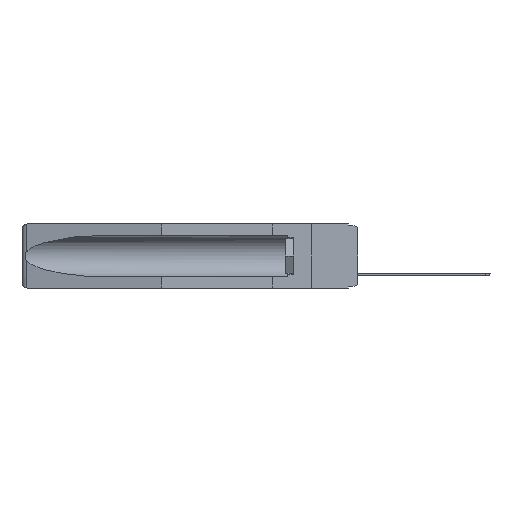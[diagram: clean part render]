
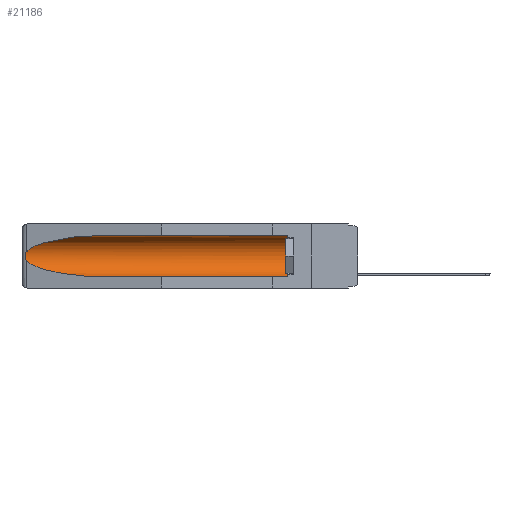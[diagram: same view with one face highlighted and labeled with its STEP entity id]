
A CAD part, left-side view. The second image highlights one B-rep face of the part: STEP entity #21186.
In plain terms, the highlighted cylindrical face has radius 2.857 mm (diameter 5.715 mm), a partial arc.
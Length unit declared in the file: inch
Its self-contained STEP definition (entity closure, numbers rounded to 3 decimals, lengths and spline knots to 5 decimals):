
#481 = CIRCLE ( 'NONE', #21289, 0.1125 ) ;
#1077 = DIRECTION ( 'NONE',  ( 0., 1., 0. ) ) ;
#1328 = DIRECTION ( 'NONE',  ( 0., 0., 1. ) ) ;
#1434 = VECTOR ( 'NONE', #1077, 39.37008 ) ;
#1686 = EDGE_CURVE ( 'NONE', #8892, #21589, #19231, .T. ) ;
#2324 = CARTESIAN_POINT ( 'NONE',  ( 0.155, 0.126, -0.284 ) ) ;
#2715 = DIRECTION ( 'NONE',  ( 0., 1., 0. ) ) ;
#2845 = CARTESIAN_POINT ( 'NONE',  ( 0.26597, 1.52961, -0.15275 ) ) ;
#3074 = CARTESIAN_POINT ( 'NONE',  ( 0.26537, 1.52718, -0.19328 ) ) ;
#3083 = CARTESIAN_POINT ( 'NONE',  ( 0.2673, 1.53269, -0.17917 ) ) ;
#3237 = EDGE_CURVE ( 'NONE', #3274, #9180, #11163, .T. ) ;
#3274 = VERTEX_POINT ( 'NONE', #3074 ) ;
#3416 = CARTESIAN_POINT ( 'NONE',  ( 0.26537, 1.52718, -0.14972 ) ) ;
#4230 = ORIENTED_EDGE ( 'NONE', *, *, #17384, .F. ) ;
#4525 = DIRECTION ( 'NONE',  ( 0., 0., 1. ) ) ;
#4943 = CYLINDRICAL_SURFACE ( 'NONE', #17287, 0.1125 ) ;
#5254 = FACE_OUTER_BOUND ( 'NONE', #5473, .T. ) ;
#5473 = EDGE_LOOP ( 'NONE', ( #9655, #9123, #10495, #4230, #18955, #6420 ) ) ;
#5537 = CARTESIAN_POINT ( 'NONE',  ( 0.155, -0.30754, -0.059 ) ) ;
#5912 = EDGE_CURVE ( 'NONE', #6770, #3274, #7760, .T. ) ;
#6420 = ORIENTED_EDGE ( 'NONE', *, *, #1686, .T. ) ;
#6770 = VERTEX_POINT ( 'NONE', #9523 ) ;
#7050 =( BOUNDED_CURVE ( )  B_SPLINE_CURVE ( 3, ( #15745, #17466, #19230, #3416 ),
 .UNSPECIFIED., .F., .F. ) 
 B_SPLINE_CURVE_WITH_KNOTS ( ( 4, 4 ),
 ( 4.71239, 6.08839 ),
 .UNSPECIFIED. ) 
 CURVE ( )  GEOMETRIC_REPRESENTATION_ITEM ( )  RATIONAL_B_SPLINE_CURVE ( ( 1., 0.848, 0.848, 1. ) ) 
 REPRESENTATION_ITEM ( '' )  );
#7760 = B_SPLINE_CURVE_WITH_KNOTS ( 'NONE', 3,
 ( #9876, #2845, #8389, #13644, #20749, #15331, #3083, #22242, #18968, #11844 ),
 .UNSPECIFIED., .F., .F.,
 ( 4, 2, 2, 2, 4 ),
 ( 0., 0.00029, 0.00058, 0.00087, 0.00117 ),
 .UNSPECIFIED. ) ;
#8104 = CARTESIAN_POINT ( 'NONE',  ( 0.155, -0.30754, -0.284 ) ) ;
#8389 = CARTESIAN_POINT ( 'NONE',  ( 0.26654, 1.53092, -0.15636 ) ) ;
#8454 = CARTESIAN_POINT ( 'NONE',  ( 0.155, 0.126, -0.1715 ) ) ;
#8892 = VERTEX_POINT ( 'NONE', #17538 ) ;
#9123 = ORIENTED_EDGE ( 'NONE', *, *, #5912, .T. ) ;
#9180 = VERTEX_POINT ( 'NONE', #16441 ) ;
#9523 = CARTESIAN_POINT ( 'NONE',  ( 0.26537, 1.52718, -0.14972 ) ) ;
#9655 = ORIENTED_EDGE ( 'NONE', *, *, #18685, .T. ) ;
#9791 = CARTESIAN_POINT ( 'NONE',  ( 0.26537, 1.52718, -0.19328 ) ) ;
#9876 = CARTESIAN_POINT ( 'NONE',  ( 0.26537, 1.52718, -0.14972 ) ) ;
#10495 = ORIENTED_EDGE ( 'NONE', *, *, #3237, .T. ) ;
#11163 =( BOUNDED_CURVE ( )  B_SPLINE_CURVE ( 3, ( #9791, #22159, #11536, #20422 ),
 .UNSPECIFIED., .F., .F. ) 
 B_SPLINE_CURVE_WITH_KNOTS ( ( 4, 4 ),
 ( 0.1948, 1.5708 ),
 .UNSPECIFIED. ) 
 CURVE ( )  GEOMETRIC_REPRESENTATION_ITEM ( )  RATIONAL_B_SPLINE_CURVE ( ( 1., 0.848, 0.848, 1. ) ) 
 REPRESENTATION_ITEM ( '' )  );
#11536 = CARTESIAN_POINT ( 'NONE',  ( 0.21114, 1.30732, -0.284 ) ) ;
#11844 = CARTESIAN_POINT ( 'NONE',  ( 0.26537, 1.52718, -0.19328 ) ) ;
#13624 = DIRECTION ( 'NONE',  ( 0., -1., 0. ) ) ;
#13644 = CARTESIAN_POINT ( 'NONE',  ( 0.2673, 1.5327, -0.16383 ) ) ;
#14283 = DIRECTION ( 'NONE',  ( 0., 1., 0. ) ) ;
#15188 = CARTESIAN_POINT ( 'NONE',  ( 0.155, 1.07973, -0.059 ) ) ;
#15331 = CARTESIAN_POINT ( 'NONE',  ( 0.2675, 1.53308, -0.17534 ) ) ;
#15745 = CARTESIAN_POINT ( 'NONE',  ( 0.155, 1.07973, -0.059 ) ) ;
#16441 = CARTESIAN_POINT ( 'NONE',  ( 0.155, 1.07973, -0.284 ) ) ;
#16454 = VECTOR ( 'NONE', #14283, 39.37008 ) ;
#17287 = AXIS2_PLACEMENT_3D ( 'NONE', #20781, #2715, #4525 ) ;
#17384 = EDGE_CURVE ( 'NONE', #23013, #9180, #22824, .T. ) ;
#17466 = CARTESIAN_POINT ( 'NONE',  ( 0.21114, 1.30732, -0.059 ) ) ;
#17538 = CARTESIAN_POINT ( 'NONE',  ( 0.155, 0.126, -0.059 ) ) ;
#18685 = EDGE_CURVE ( 'NONE', #21589, #6770, #7050, .T. ) ;
#18955 = ORIENTED_EDGE ( 'NONE', *, *, #20508, .T. ) ;
#18968 = CARTESIAN_POINT ( 'NONE',  ( 0.26597, 1.5296, -0.19026 ) ) ;
#19230 = CARTESIAN_POINT ( 'NONE',  ( 0.25451, 1.48313, -0.09465 ) ) ;
#19231 = LINE ( 'NONE', #5537, #16454 ) ;
#20422 = CARTESIAN_POINT ( 'NONE',  ( 0.155, 1.07973, -0.284 ) ) ;
#20508 = EDGE_CURVE ( 'NONE', #23013, #8892, #481, .T. ) ;
#20749 = CARTESIAN_POINT ( 'NONE',  ( 0.2675, 1.53308, -0.16763 ) ) ;
#20781 = CARTESIAN_POINT ( 'NONE',  ( 0.155, -0.30754, -0.1715 ) ) ;
#21186 = ADVANCED_FACE ( 'NONE', ( #5254 ), #4943, .F. ) ;
#21289 = AXIS2_PLACEMENT_3D ( 'NONE', #8454, #13624, #1328 ) ;
#21589 = VERTEX_POINT ( 'NONE', #15188 ) ;
#22159 = CARTESIAN_POINT ( 'NONE',  ( 0.25451, 1.48313, -0.24835 ) ) ;
#22242 = CARTESIAN_POINT ( 'NONE',  ( 0.26655, 1.53094, -0.18657 ) ) ;
#22824 = LINE ( 'NONE', #8104, #1434 ) ;
#23013 = VERTEX_POINT ( 'NONE', #2324 ) ;
